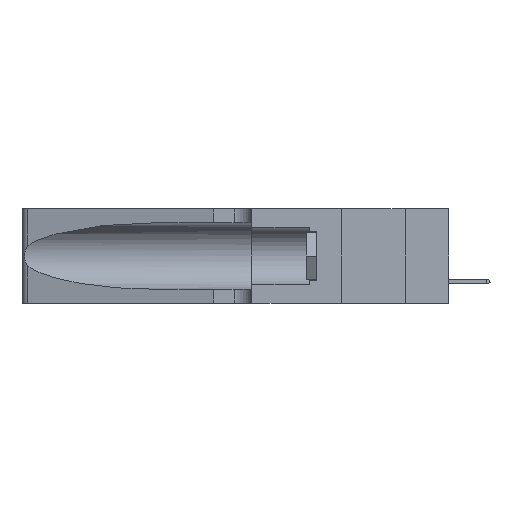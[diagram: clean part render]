
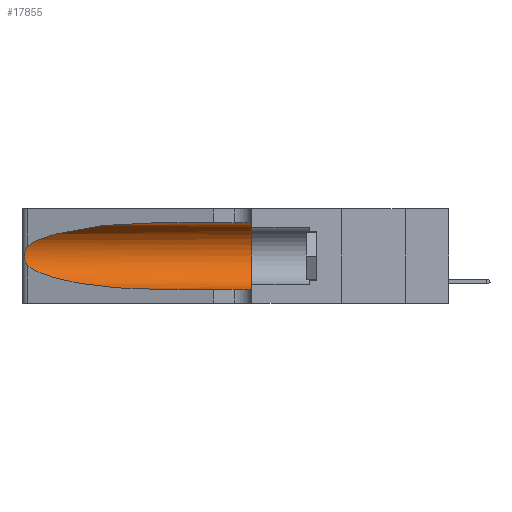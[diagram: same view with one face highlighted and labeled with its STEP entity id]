
A CAD part, left-side view. The second image highlights one B-rep face of the part: STEP entity #17855.
In plain terms, the highlighted cylindrical face has radius 3.308 mm (diameter 6.617 mm), a partial arc.
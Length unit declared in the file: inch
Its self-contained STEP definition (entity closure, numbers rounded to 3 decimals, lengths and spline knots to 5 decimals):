
#1920 = CARTESIAN_POINT ( 'NONE',  ( 0.18966, 0.96281, 0.05475 ) ) ;
#2032 = CARTESIAN_POINT ( 'NONE',  ( 0.1305, 0.72297, 0.31525 ) ) ;
#2212 = ORIENTED_EDGE ( 'NONE', *, *, #8784, .T. ) ;
#2222 = FACE_OUTER_BOUND ( 'NONE', #17480, .T. ) ;
#2594 = CARTESIAN_POINT ( 'NONE',  ( 0.18966, 0.96281, 0.31525 ) ) ;
#2788 = AXIS2_PLACEMENT_3D ( 'NONE', #17141, #19300, #23613 ) ;
#3254 = CIRCLE ( 'NONE', #2788, 0.13025 ) ;
#3440 = CARTESIAN_POINT ( 'NONE',  ( 0.25787, 1.23484, 0.2124 ) ) ;
#3510 = VERTEX_POINT ( 'NONE', #18189 ) ;
#3588 = VERTEX_POINT ( 'NONE', #11683 ) ;
#3808 = CARTESIAN_POINT ( 'NONE',  ( 0.25487, 1.22718, 0.14631 ) ) ;
#5180 = CARTESIAN_POINT ( 'NONE',  ( 0.1305, 0.35, 0.31525 ) ) ;
#5530 = ORIENTED_EDGE ( 'NONE', *, *, #10867, .F. ) ;
#5751 = DIRECTION ( 'NONE',  ( 0., -1., 0. ) ) ;
#6133 = CARTESIAN_POINT ( 'NONE',  ( 0.1305, 0.72297, 0.05475 ) ) ;
#6314 = EDGE_CURVE ( 'NONE', #22214, #3510, #16565, .T. ) ;
#6321 = CARTESIAN_POINT ( 'NONE',  ( 0.2373, 1.15595, 0.08982 ) ) ;
#8149 = CARTESIAN_POINT ( 'NONE',  ( 0.26075, 1.23896, 0.178 ) ) ;
#8498 = CARTESIAN_POINT ( 'NONE',  ( 0.25487, 1.22718, 0.22369 ) ) ;
#8681 = ORIENTED_EDGE ( 'NONE', *, *, #22500, .T. ) ;
#8784 = EDGE_CURVE ( 'NONE', #18353, #3588, #19235, .T. ) ;
#9272 = EDGE_CURVE ( 'NONE', #19621, #21408, #10449, .T. ) ;
#10325 = CARTESIAN_POINT ( 'NONE',  ( 0.25487, 1.22718, 0.22369 ) ) ;
#10449 = LINE ( 'NONE', #24181, #27583 ) ;
#10867 = EDGE_CURVE ( 'NONE', #21408, #3588, #3254, .T. ) ;
#11541 =( BOUNDED_CURVE ( )  B_SPLINE_CURVE ( 3, ( #2032, #2594, #19391, #13891 ),
 .UNSPECIFIED., .F., .T. ) 
 B_SPLINE_CURVE_WITH_KNOTS ( ( 4, 4 ),
 ( 1.5708, 2.84003 ),
 .UNSPECIFIED. ) 
 CURVE ( )  GEOMETRIC_REPRESENTATION_ITEM ( )  RATIONAL_B_SPLINE_CURVE ( ( 1., 0.87, 0.87, 1. ) ) 
 REPRESENTATION_ITEM ( '' )  );
#11683 = CARTESIAN_POINT ( 'NONE',  ( 0.1305, 0.35, 0.05475 ) ) ;
#12198 = CARTESIAN_POINT ( 'NONE',  ( 0.25789, 1.23486, 0.15765 ) ) ;
#12229 = CYLINDRICAL_SURFACE ( 'NONE', #21340, 0.13025 ) ;
#12547 = ORIENTED_EDGE ( 'NONE', *, *, #9272, .F. ) ;
#13891 = CARTESIAN_POINT ( 'NONE',  ( 0.25487, 1.22718, 0.22369 ) ) ;
#14285 = CARTESIAN_POINT ( 'NONE',  ( 0.25639, 1.23186, 0.15144 ) ) ;
#14349 = CARTESIAN_POINT ( 'NONE',  ( 0.1305, 0.72297, 0.05475 ) ) ;
#14464 = CARTESIAN_POINT ( 'NONE',  ( 0.25856, 1.23593, 0.16098 ) ) ;
#15826 = DIRECTION ( 'NONE',  ( 0., -1., 0. ) ) ;
#16475 = CARTESIAN_POINT ( 'NONE',  ( 0.26018, 1.23835, 0.19895 ) ) ;
#16565 = B_SPLINE_CURVE_WITH_KNOTS ( 'NONE', 3,
 ( #10325, #16764, #25283, #3440, #23038, #16475, #18924, #8149, #18544, #14464, #12198, #14285, #27229, #3808 ),
 .UNSPECIFIED., .F., .F.,
 ( 4, 2, 2, 2, 2, 2, 4 ),
 ( 0., 0.00027, 0.00053, 0.00107, 0.0016, 0.00187, 0.00214 ),
 .UNSPECIFIED. ) ;
#16764 = CARTESIAN_POINT ( 'NONE',  ( 0.25555, 1.22994, 0.2215 ) ) ;
#16829 = ORIENTED_EDGE ( 'NONE', *, *, #18603, .T. ) ;
#17141 = CARTESIAN_POINT ( 'NONE',  ( 0.1305, 0.35, 0.185 ) ) ;
#17480 = EDGE_LOOP ( 'NONE', ( #16829, #22480, #8681, #2212, #5530, #12547 ) ) ;
#17855 = ADVANCED_FACE ( 'NONE', ( #2222 ), #12229, .F. ) ;
#18189 = CARTESIAN_POINT ( 'NONE',  ( 0.25487, 1.22718, 0.14631 ) ) ;
#18353 = VERTEX_POINT ( 'NONE', #14349 ) ;
#18544 = CARTESIAN_POINT ( 'NONE',  ( 0.26017, 1.23833, 0.17102 ) ) ;
#18547 = VECTOR ( 'NONE', #19553, 39.37008 ) ;
#18603 = EDGE_CURVE ( 'NONE', #19621, #22214, #11541, .T. ) ;
#18681 = CARTESIAN_POINT ( 'NONE',  ( 0.1305, 1.61858, 0.185 ) ) ;
#18924 = CARTESIAN_POINT ( 'NONE',  ( 0.26075, 1.23896, 0.19203 ) ) ;
#19235 = LINE ( 'NONE', #25081, #18547 ) ;
#19300 = DIRECTION ( 'NONE',  ( 0., 1., 0. ) ) ;
#19391 = CARTESIAN_POINT ( 'NONE',  ( 0.2373, 1.15595, 0.28018 ) ) ;
#19490 = CARTESIAN_POINT ( 'NONE',  ( 0.1305, 0.72297, 0.31525 ) ) ;
#19553 = DIRECTION ( 'NONE',  ( 0., -1., 0. ) ) ;
#19621 = VERTEX_POINT ( 'NONE', #19490 ) ;
#21340 = AXIS2_PLACEMENT_3D ( 'NONE', #18681, #5751, #27533 ) ;
#21408 = VERTEX_POINT ( 'NONE', #5180 ) ;
#22214 = VERTEX_POINT ( 'NONE', #8498 ) ;
#22480 = ORIENTED_EDGE ( 'NONE', *, *, #6314, .T. ) ;
#22500 = EDGE_CURVE ( 'NONE', #3510, #18353, #24462, .T. ) ;
#23038 = CARTESIAN_POINT ( 'NONE',  ( 0.25854, 1.2359, 0.20912 ) ) ;
#23613 = DIRECTION ( 'NONE',  ( 0., 0., 1. ) ) ;
#24181 = CARTESIAN_POINT ( 'NONE',  ( 0.1305, 1.61858, 0.31525 ) ) ;
#24462 =( BOUNDED_CURVE ( )  B_SPLINE_CURVE ( 3, ( #25034, #6321, #1920, #6133 ),
 .UNSPECIFIED., .F., .T. ) 
 B_SPLINE_CURVE_WITH_KNOTS ( ( 4, 4 ),
 ( 3.44316, 4.71239 ),
 .UNSPECIFIED. ) 
 CURVE ( )  GEOMETRIC_REPRESENTATION_ITEM ( )  RATIONAL_B_SPLINE_CURVE ( ( 1., 0.87, 0.87, 1. ) ) 
 REPRESENTATION_ITEM ( '' )  );
#25034 = CARTESIAN_POINT ( 'NONE',  ( 0.25487, 1.22718, 0.14631 ) ) ;
#25081 = CARTESIAN_POINT ( 'NONE',  ( 0.1305, 1.61858, 0.05475 ) ) ;
#25283 = CARTESIAN_POINT ( 'NONE',  ( 0.25639, 1.23184, 0.21858 ) ) ;
#27229 = CARTESIAN_POINT ( 'NONE',  ( 0.25555, 1.22993, 0.14849 ) ) ;
#27533 = DIRECTION ( 'NONE',  ( 0., 0., -1. ) ) ;
#27583 = VECTOR ( 'NONE', #15826, 39.37008 ) ;
